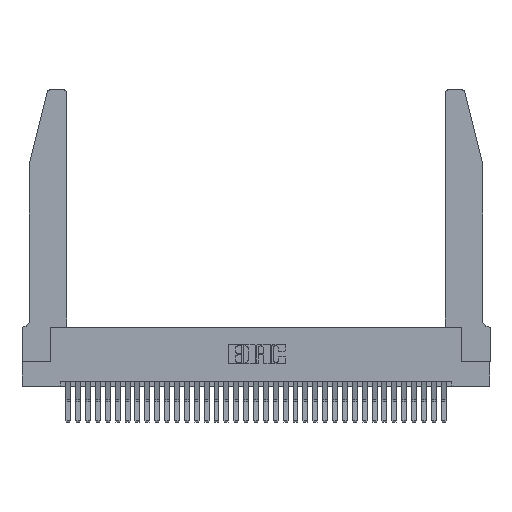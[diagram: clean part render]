
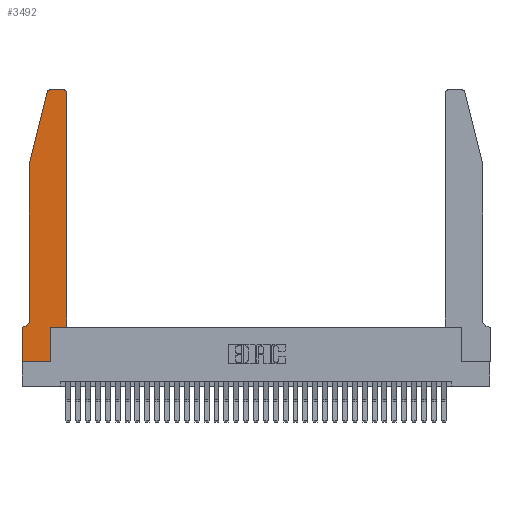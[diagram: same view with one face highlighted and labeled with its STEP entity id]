
A CAD part, top view. The second image highlights one B-rep face of the part: STEP entity #3492.
In plain terms, the highlighted planar face has unit normal (0, 0, 1).
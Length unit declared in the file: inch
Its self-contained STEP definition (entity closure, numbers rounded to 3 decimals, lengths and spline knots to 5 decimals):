
#201 = VERTEX_POINT ( 'NONE', #3399 ) ;
#211 = CIRCLE ( 'NONE', #4844, 0.03 ) ;
#1281 = CARTESIAN_POINT ( 'NONE',  ( 0.4505, 0.35, 0.37 ) ) ;
#1773 = AXIS2_PLACEMENT_3D ( 'NONE', #15661, #18208, #10117 ) ;
#1975 = DIRECTION ( 'NONE',  ( 0., 0., -1. ) ) ;
#2376 = CARTESIAN_POINT ( 'NONE',  ( 0., 0., 0.37 ) ) ;
#2621 = EDGE_CURVE ( 'NONE', #20850, #2788, #22939, .T. ) ;
#2751 = VERTEX_POINT ( 'NONE', #16097 ) ;
#2788 = VERTEX_POINT ( 'NONE', #24739 ) ;
#3115 = VECTOR ( 'NONE', #15735, 39.37008 ) ;
#3399 = CARTESIAN_POINT ( 'NONE',  ( 0.0755, 0.42, 0.37 ) ) ;
#3492 = ADVANCED_FACE ( 'NONE', ( #26796 ), #25193, .T. ) ;
#3846 = CARTESIAN_POINT ( 'NONE',  ( 0.0755, 2., 0.37 ) ) ;
#4482 = LINE ( 'NONE', #22873, #33111 ) ;
#4844 = AXIS2_PLACEMENT_3D ( 'NONE', #27036, #18597, #10523 ) ;
#4984 = ORIENTED_EDGE ( 'NONE', *, *, #9780, .T. ) ;
#5070 = LINE ( 'NONE', #7337, #23669 ) ;
#5242 = VECTOR ( 'NONE', #16247, 39.37008 ) ;
#5371 = EDGE_CURVE ( 'NONE', #11590, #201, #13952, .T. ) ;
#5619 = VERTEX_POINT ( 'NONE', #10738 ) ;
#6134 = VECTOR ( 'NONE', #15691, 39.37008 ) ;
#6178 = DIRECTION ( 'NONE',  ( -1., 0., 0. ) ) ;
#6869 = ORIENTED_EDGE ( 'NONE', *, *, #11812, .T. ) ;
#7337 = CARTESIAN_POINT ( 'NONE',  ( 0.2605, 2.75, 0.37 ) ) ;
#7378 = DIRECTION ( 'NONE',  ( -1., 0., 0. ) ) ;
#7463 = CIRCLE ( 'NONE', #1773, 0.03 ) ;
#7499 = EDGE_CURVE ( 'NONE', #2751, #8352, #5070, .T. ) ;
#7994 = LINE ( 'NONE', #34931, #3115 ) ;
#8165 = VECTOR ( 'NONE', #17398, 39.37008 ) ;
#8352 = VERTEX_POINT ( 'NONE', #18185 ) ;
#8573 = EDGE_CURVE ( 'NONE', #2788, #2751, #211, .T. ) ;
#9780 = EDGE_CURVE ( 'NONE', #23613, #30403, #4482, .T. ) ;
#10117 = DIRECTION ( 'NONE',  ( 1., 0., 0. ) ) ;
#10523 = DIRECTION ( 'NONE',  ( 1., 0., 0. ) ) ;
#10632 = CARTESIAN_POINT ( 'NONE',  ( 0.25487, 2.72718, 0.37 ) ) ;
#10738 = CARTESIAN_POINT ( 'NONE',  ( 0., 0., 0.37 ) ) ;
#11046 = LINE ( 'NONE', #31938, #31276 ) ;
#11281 = EDGE_CURVE ( 'NONE', #201, #23613, #17953, .T. ) ;
#11590 = VERTEX_POINT ( 'NONE', #3846 ) ;
#11812 = EDGE_CURVE ( 'NONE', #30150, #20850, #11046, .T. ) ;
#12058 = EDGE_CURVE ( 'NONE', #32991, #30150, #7994, .T. ) ;
#12122 = EDGE_CURVE ( 'NONE', #16102, #11590, #31707, .T. ) ;
#12758 = ORIENTED_EDGE ( 'NONE', *, *, #18090, .T. ) ;
#12902 = AXIS2_PLACEMENT_3D ( 'NONE', #31065, #31185, #28510 ) ;
#13087 = ORIENTED_EDGE ( 'NONE', *, *, #14274, .T. ) ;
#13706 = DIRECTION ( 'NONE',  ( 1., 0., 0. ) ) ;
#13855 = ORIENTED_EDGE ( 'NONE', *, *, #8573, .T. ) ;
#13952 = LINE ( 'NONE', #25453, #16910 ) ;
#14083 = ORIENTED_EDGE ( 'NONE', *, *, #2621, .T. ) ;
#14274 = EDGE_CURVE ( 'NONE', #5619, #32991, #32045, .T. ) ;
#14773 = CARTESIAN_POINT ( 'NONE',  ( 0., 0.35, 0.37 ) ) ;
#15661 = CARTESIAN_POINT ( 'NONE',  ( 0.284, 2.72, 0.37 ) ) ;
#15687 = ORIENTED_EDGE ( 'NONE', *, *, #16235, .T. ) ;
#15691 = DIRECTION ( 'NONE',  ( -0.239, -0.971, 0. ) ) ;
#15735 = DIRECTION ( 'NONE',  ( 0., 1., 0. ) ) ;
#16097 = CARTESIAN_POINT ( 'NONE',  ( 0.4205, 2.75, 0.37 ) ) ;
#16102 = VERTEX_POINT ( 'NONE', #10632 ) ;
#16235 = EDGE_CURVE ( 'NONE', #30403, #5619, #31026, .T. ) ;
#16247 = DIRECTION ( 'NONE',  ( 1., 0., 0. ) ) ;
#16910 = VECTOR ( 'NONE', #34227, 39.37008 ) ;
#17395 = ORIENTED_EDGE ( 'NONE', *, *, #7499, .T. ) ;
#17398 = DIRECTION ( 'NONE',  ( 0., -1., 0. ) ) ;
#17503 = CARTESIAN_POINT ( 'NONE',  ( 0.2865, 0., 0.37 ) ) ;
#17769 = ORIENTED_EDGE ( 'NONE', *, *, #12122, .T. ) ;
#17953 = CIRCLE ( 'NONE', #19349, 0.07 ) ;
#18090 = EDGE_CURVE ( 'NONE', #8352, #16102, #7463, .T. ) ;
#18185 = CARTESIAN_POINT ( 'NONE',  ( 0.284, 2.75, 0.37 ) ) ;
#18208 = DIRECTION ( 'NONE',  ( 0., 0., 1. ) ) ;
#18400 = CARTESIAN_POINT ( 'NONE',  ( 0.0055, 0.42, 0.37 ) ) ;
#18597 = DIRECTION ( 'NONE',  ( 0., 0., 1. ) ) ;
#19349 = AXIS2_PLACEMENT_3D ( 'NONE', #18400, #1975, #7378 ) ;
#20850 = VERTEX_POINT ( 'NONE', #33283 ) ;
#22019 = EDGE_LOOP ( 'NONE', ( #17395, #12758, #17769, #27128, #31805, #4984, #15687, #13087, #27510, #6869, #14083, #13855 ) ) ;
#22485 = CARTESIAN_POINT ( 'NONE',  ( 0.0755, 2., 0.37 ) ) ;
#22784 = CARTESIAN_POINT ( 'NONE',  ( 0.2865, 0.35, 0.37 ) ) ;
#22873 = CARTESIAN_POINT ( 'NONE',  ( 0.0755, 0.35, 0.37 ) ) ;
#22939 = LINE ( 'NONE', #1281, #23389 ) ;
#23389 = VECTOR ( 'NONE', #23665, 39.37008 ) ;
#23613 = VERTEX_POINT ( 'NONE', #34944 ) ;
#23665 = DIRECTION ( 'NONE',  ( 0., 1., 0. ) ) ;
#23669 = VECTOR ( 'NONE', #30550, 39.37008 ) ;
#23743 = CARTESIAN_POINT ( 'NONE',  ( 0., 0., 0.37 ) ) ;
#24739 = CARTESIAN_POINT ( 'NONE',  ( 0.4505, 2.72, 0.37 ) ) ;
#25193 = PLANE ( 'NONE',  #12902 ) ;
#25453 = CARTESIAN_POINT ( 'NONE',  ( 0.0755, 2., 0.37 ) ) ;
#26796 = FACE_OUTER_BOUND ( 'NONE', #22019, .T. ) ;
#27036 = CARTESIAN_POINT ( 'NONE',  ( 0.4205, 2.72, 0.37 ) ) ;
#27128 = ORIENTED_EDGE ( 'NONE', *, *, #5371, .T. ) ;
#27510 = ORIENTED_EDGE ( 'NONE', *, *, #12058, .T. ) ;
#28510 = DIRECTION ( 'NONE',  ( 1., 0., 0. ) ) ;
#30150 = VERTEX_POINT ( 'NONE', #22784 ) ;
#30403 = VERTEX_POINT ( 'NONE', #14773 ) ;
#30550 = DIRECTION ( 'NONE',  ( -1., 0., 0. ) ) ;
#31026 = LINE ( 'NONE', #23743, #8165 ) ;
#31065 = CARTESIAN_POINT ( 'NONE',  ( 0., 0.35, 0.37 ) ) ;
#31185 = DIRECTION ( 'NONE',  ( 0., 0., 1. ) ) ;
#31276 = VECTOR ( 'NONE', #13706, 39.37008 ) ;
#31707 = LINE ( 'NONE', #22485, #6134 ) ;
#31805 = ORIENTED_EDGE ( 'NONE', *, *, #11281, .T. ) ;
#31938 = CARTESIAN_POINT ( 'NONE',  ( 0.4505, 0.35, 0.37 ) ) ;
#32045 = LINE ( 'NONE', #2376, #5242 ) ;
#32991 = VERTEX_POINT ( 'NONE', #17503 ) ;
#33111 = VECTOR ( 'NONE', #6178, 39.37008 ) ;
#33283 = CARTESIAN_POINT ( 'NONE',  ( 0.4505, 0.35, 0.37 ) ) ;
#34227 = DIRECTION ( 'NONE',  ( 0., -1., 0. ) ) ;
#34931 = CARTESIAN_POINT ( 'NONE',  ( 0.2865, 0.35, 0.37 ) ) ;
#34944 = CARTESIAN_POINT ( 'NONE',  ( 0.0055, 0.35, 0.37 ) ) ;
